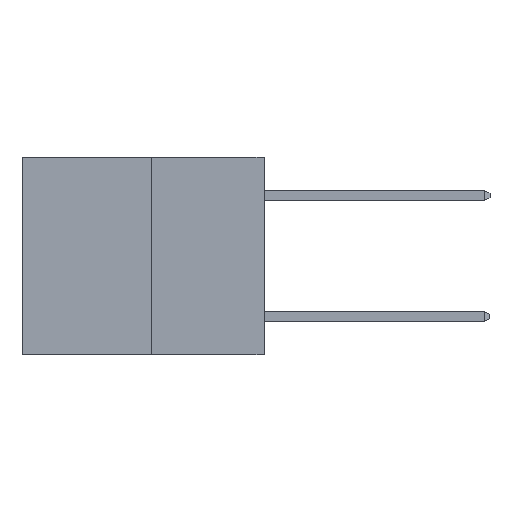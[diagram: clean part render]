
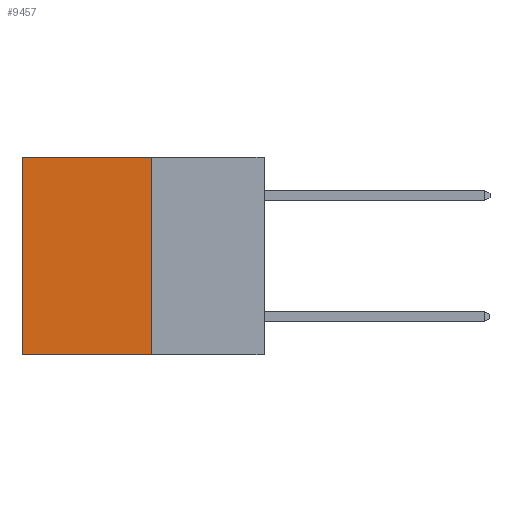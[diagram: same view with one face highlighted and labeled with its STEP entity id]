
A CAD part, left-side view. The second image highlights one B-rep face of the part: STEP entity #9457.
In plain terms, the highlighted planar face has unit normal (-1, 0, 0).
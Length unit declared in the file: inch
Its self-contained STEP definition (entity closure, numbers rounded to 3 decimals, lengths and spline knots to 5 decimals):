
#110 = VECTOR ( 'NONE', #9826, 39.37008 ) ;
#1314 = EDGE_LOOP ( 'NONE', ( #6004, #15879, #20223, #17944 ) ) ;
#1880 = LINE ( 'NONE', #17498, #3121 ) ;
#2573 = LINE ( 'NONE', #3093, #15627 ) ;
#3093 = CARTESIAN_POINT ( 'NONE',  ( 0.3165, 0.28, -0.49 ) ) ;
#3121 = VECTOR ( 'NONE', #4768, 39.37008 ) ;
#3147 = AXIS2_PLACEMENT_3D ( 'NONE', #7314, #7246, #5828 ) ;
#4768 = DIRECTION ( 'NONE',  ( 0., 0., -1. ) ) ;
#4795 = LINE ( 'NONE', #8962, #10457 ) ;
#4834 = VERTEX_POINT ( 'NONE', #8303 ) ;
#5828 = DIRECTION ( 'NONE',  ( 0., 0., -1. ) ) ;
#6004 = ORIENTED_EDGE ( 'NONE', *, *, #14518, .T. ) ;
#6948 = VERTEX_POINT ( 'NONE', #10362 ) ;
#7246 = DIRECTION ( 'NONE',  ( 1., 0., 0. ) ) ;
#7314 = CARTESIAN_POINT ( 'NONE',  ( 0.3165, 0.28, -0.49 ) ) ;
#8303 = CARTESIAN_POINT ( 'NONE',  ( 0.3165, 0.6, -0.49 ) ) ;
#8413 = VERTEX_POINT ( 'NONE', #12133 ) ;
#8962 = CARTESIAN_POINT ( 'NONE',  ( 0.3165, 0.28, -0.49 ) ) ;
#9457 = ADVANCED_FACE ( 'NONE', ( #11800 ), #16982, .F. ) ;
#9681 = LINE ( 'NONE', #15970, #110 ) ;
#9826 = DIRECTION ( 'NONE',  ( 0., 1., 0. ) ) ;
#10362 = CARTESIAN_POINT ( 'NONE',  ( 0.3165, 0.28, 0. ) ) ;
#10457 = VECTOR ( 'NONE', #10694, 39.37008 ) ;
#10694 = DIRECTION ( 'NONE',  ( 0., 0., -1. ) ) ;
#11800 = FACE_OUTER_BOUND ( 'NONE', #1314, .T. ) ;
#12133 = CARTESIAN_POINT ( 'NONE',  ( 0.3165, 0.6, 0. ) ) ;
#12540 = DIRECTION ( 'NONE',  ( 0., 1., 0. ) ) ;
#14095 = CARTESIAN_POINT ( 'NONE',  ( 0.3165, 0.28, -0.49 ) ) ;
#14518 = EDGE_CURVE ( 'NONE', #8413, #4834, #1880, .T. ) ;
#15193 = EDGE_CURVE ( 'NONE', #6948, #19655, #4795, .T. ) ;
#15369 = EDGE_CURVE ( 'NONE', #19655, #4834, #2573, .T. ) ;
#15627 = VECTOR ( 'NONE', #12540, 39.37008 ) ;
#15879 = ORIENTED_EDGE ( 'NONE', *, *, #15369, .F. ) ;
#15970 = CARTESIAN_POINT ( 'NONE',  ( 0.3165, 0.28, 0. ) ) ;
#16982 = PLANE ( 'NONE',  #3147 ) ;
#17498 = CARTESIAN_POINT ( 'NONE',  ( 0.3165, 0.6, -0.49 ) ) ;
#17944 = ORIENTED_EDGE ( 'NONE', *, *, #20258, .T. ) ;
#19655 = VERTEX_POINT ( 'NONE', #14095 ) ;
#20223 = ORIENTED_EDGE ( 'NONE', *, *, #15193, .F. ) ;
#20258 = EDGE_CURVE ( 'NONE', #6948, #8413, #9681, .T. ) ;
